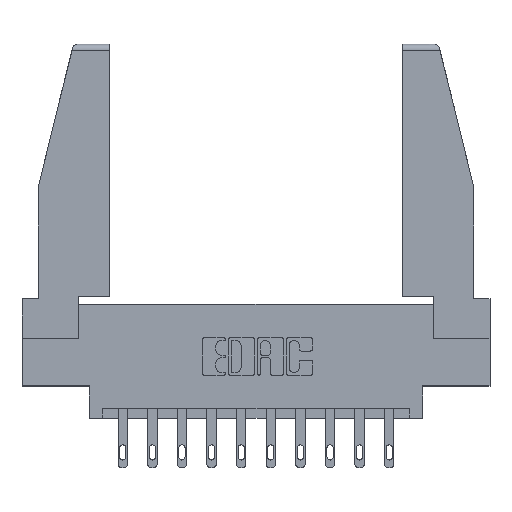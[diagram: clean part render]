
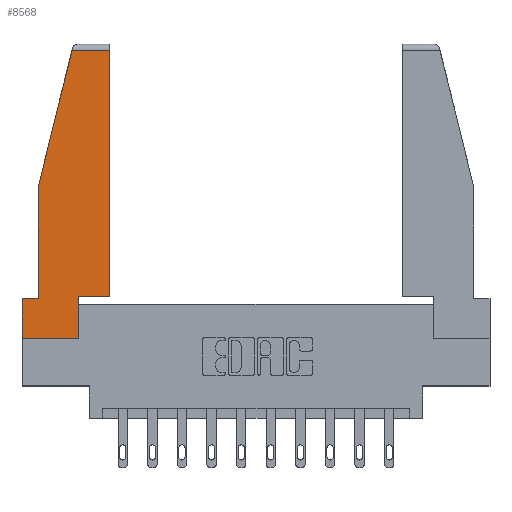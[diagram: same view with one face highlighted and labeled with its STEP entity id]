
A CAD part, top view. The second image highlights one B-rep face of the part: STEP entity #8568.
In plain terms, the highlighted planar face has unit normal (0, 0, 1).
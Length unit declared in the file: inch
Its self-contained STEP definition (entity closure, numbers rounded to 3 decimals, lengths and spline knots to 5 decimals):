
#61 = VECTOR ( 'NONE', #3460, 39.37008 ) ;
#200 = LINE ( 'NONE', #2220, #5903 ) ;
#529 = DIRECTION ( 'NONE',  ( 0., -1., 0. ) ) ;
#535 = VERTEX_POINT ( 'NONE', #12174 ) ;
#668 = ORIENTED_EDGE ( 'NONE', *, *, #14208, .T. ) ;
#1061 = CARTESIAN_POINT ( 'NONE',  ( 0., 0., 0. ) ) ;
#1241 = CARTESIAN_POINT ( 'NONE',  ( 0., 0.21, 0. ) ) ;
#1322 = CARTESIAN_POINT ( 'NONE',  ( 0., 0.21, 0. ) ) ;
#1355 = LINE ( 'NONE', #1241, #11624 ) ;
#1505 = CARTESIAN_POINT ( 'NONE',  ( 0.271, 1.55, 0. ) ) ;
#1766 = VERTEX_POINT ( 'NONE', #7154 ) ;
#1926 = VERTEX_POINT ( 'NONE', #7263 ) ;
#2103 = LINE ( 'NONE', #1505, #3350 ) ;
#2160 = DIRECTION ( 'NONE',  ( 1., 0., 0. ) ) ;
#2220 = CARTESIAN_POINT ( 'NONE',  ( 0.297, 0.223, 0. ) ) ;
#2261 = PLANE ( 'NONE',  #9725 ) ;
#3350 = VECTOR ( 'NONE', #11405, 39.37008 ) ;
#3369 = LINE ( 'NONE', #10548, #11392 ) ;
#3460 = DIRECTION ( 'NONE',  ( 0., 1., 0. ) ) ;
#3805 = DIRECTION ( 'NONE',  ( 0., -1., 0. ) ) ;
#4083 = ORIENTED_EDGE ( 'NONE', *, *, #4657, .T. ) ;
#4437 = FACE_OUTER_BOUND ( 'NONE', #5220, .T. ) ;
#4513 = LINE ( 'NONE', #1322, #4681 ) ;
#4597 = EDGE_CURVE ( 'NONE', #12292, #9655, #9065, .T. ) ;
#4657 = EDGE_CURVE ( 'NONE', #13616, #9455, #2103, .T. ) ;
#4681 = VECTOR ( 'NONE', #529, 39.37008 ) ;
#4840 = CARTESIAN_POINT ( 'NONE',  ( 0.086, 0.8, 0. ) ) ;
#5220 = EDGE_LOOP ( 'NONE', ( #6073, #6890, #4083, #668, #5562, #13472, #13943, #9770, #9828 ) ) ;
#5427 = DIRECTION ( 'NONE',  ( 1., 0., 0. ) ) ;
#5562 = ORIENTED_EDGE ( 'NONE', *, *, #7837, .T. ) ;
#5709 = EDGE_CURVE ( 'NONE', #1926, #13616, #9052, .T. ) ;
#5755 = CARTESIAN_POINT ( 'NONE',  ( 0., 0.21, 0. ) ) ;
#5845 = LINE ( 'NONE', #1061, #9846 ) ;
#5903 = VECTOR ( 'NONE', #5427, 39.37008 ) ;
#6044 = VERTEX_POINT ( 'NONE', #13786 ) ;
#6073 = ORIENTED_EDGE ( 'NONE', *, *, #7632, .T. ) ;
#6368 = EDGE_CURVE ( 'NONE', #9655, #6044, #200, .T. ) ;
#6571 = EDGE_CURVE ( 'NONE', #12785, #1766, #4513, .T. ) ;
#6732 = CARTESIAN_POINT ( 'NONE',  ( 0., 0., 0. ) ) ;
#6890 = ORIENTED_EDGE ( 'NONE', *, *, #5709, .T. ) ;
#7041 = CARTESIAN_POINT ( 'NONE',  ( 0., 1.52, 0. ) ) ;
#7154 = CARTESIAN_POINT ( 'NONE',  ( 0., 0., 0. ) ) ;
#7263 = CARTESIAN_POINT ( 'NONE',  ( 0.461, 1.52, 0. ) ) ;
#7632 = EDGE_CURVE ( 'NONE', #6044, #1926, #9159, .T. ) ;
#7837 = EDGE_CURVE ( 'NONE', #535, #12785, #1355, .T. ) ;
#7981 = VECTOR ( 'NONE', #11701, 39.37008 ) ;
#8045 = CARTESIAN_POINT ( 'NONE',  ( 0.2636, 1.52, 0. ) ) ;
#8555 = EDGE_CURVE ( 'NONE', #1766, #12292, #5845, .T. ) ;
#8568 = ADVANCED_FACE ( 'NONE', ( #4437 ), #2261, .T. ) ;
#8802 = DIRECTION ( 'NONE',  ( 0., 0., 1. ) ) ;
#8995 = VECTOR ( 'NONE', #12792, 39.37008 ) ;
#9052 = LINE ( 'NONE', #7041, #7981 ) ;
#9065 = LINE ( 'NONE', #13409, #61 ) ;
#9159 = LINE ( 'NONE', #11620, #8995 ) ;
#9455 = VERTEX_POINT ( 'NONE', #4840 ) ;
#9655 = VERTEX_POINT ( 'NONE', #14031 ) ;
#9725 = AXIS2_PLACEMENT_3D ( 'NONE', #6732, #8802, #2160 ) ;
#9770 = ORIENTED_EDGE ( 'NONE', *, *, #4597, .T. ) ;
#9828 = ORIENTED_EDGE ( 'NONE', *, *, #6368, .T. ) ;
#9846 = VECTOR ( 'NONE', #12262, 39.37008 ) ;
#10548 = CARTESIAN_POINT ( 'NONE',  ( 0.086, 0.8, 0. ) ) ;
#11392 = VECTOR ( 'NONE', #3805, 39.37008 ) ;
#11405 = DIRECTION ( 'NONE',  ( -0.239, -0.971, 0. ) ) ;
#11620 = CARTESIAN_POINT ( 'NONE',  ( 0.461, 0.223, 0. ) ) ;
#11624 = VECTOR ( 'NONE', #12351, 39.37008 ) ;
#11701 = DIRECTION ( 'NONE',  ( -1., 0., 0. ) ) ;
#12174 = CARTESIAN_POINT ( 'NONE',  ( 0.086, 0.21, 0. ) ) ;
#12262 = DIRECTION ( 'NONE',  ( 1., 0., 0. ) ) ;
#12292 = VERTEX_POINT ( 'NONE', #13668 ) ;
#12351 = DIRECTION ( 'NONE',  ( -1., 0., 0. ) ) ;
#12785 = VERTEX_POINT ( 'NONE', #5755 ) ;
#12792 = DIRECTION ( 'NONE',  ( 0., 1., 0. ) ) ;
#13409 = CARTESIAN_POINT ( 'NONE',  ( 0.297, 0., 0. ) ) ;
#13472 = ORIENTED_EDGE ( 'NONE', *, *, #6571, .T. ) ;
#13616 = VERTEX_POINT ( 'NONE', #8045 ) ;
#13668 = CARTESIAN_POINT ( 'NONE',  ( 0.297, 0., 0. ) ) ;
#13786 = CARTESIAN_POINT ( 'NONE',  ( 0.461, 0.223, 0. ) ) ;
#13943 = ORIENTED_EDGE ( 'NONE', *, *, #8555, .T. ) ;
#14031 = CARTESIAN_POINT ( 'NONE',  ( 0.297, 0.223, 0. ) ) ;
#14208 = EDGE_CURVE ( 'NONE', #9455, #535, #3369, .T. ) ;
